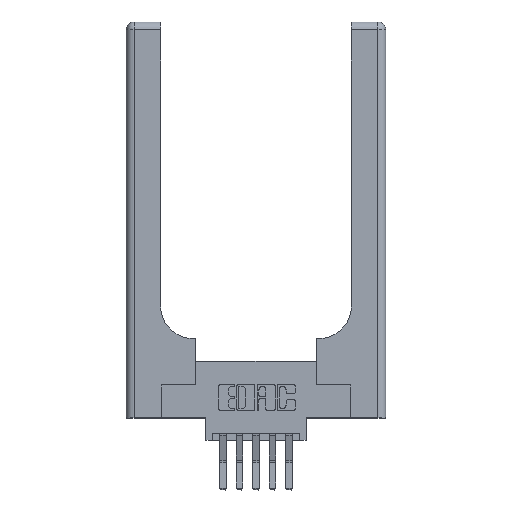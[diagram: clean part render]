
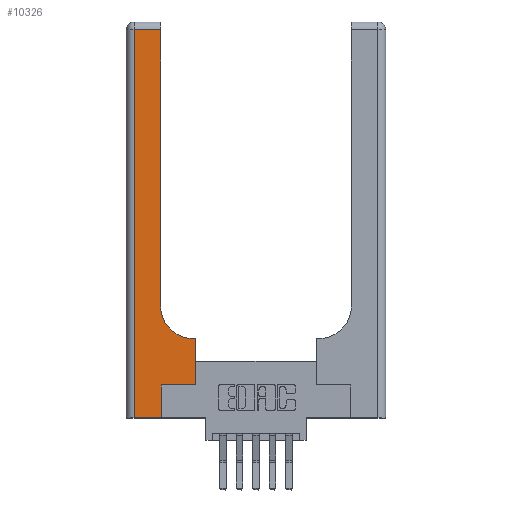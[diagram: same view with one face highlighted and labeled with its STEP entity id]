
A CAD part, top view. The second image highlights one B-rep face of the part: STEP entity #10326.
In plain terms, the highlighted planar face has unit normal (0, 0, 1).
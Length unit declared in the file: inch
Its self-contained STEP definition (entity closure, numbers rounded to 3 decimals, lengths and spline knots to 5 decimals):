
#12 = LINE ( 'NONE', #1932, #660 ) ;
#51 = CARTESIAN_POINT ( 'NONE',  ( 0., 3., 0.37 ) ) ;
#212 = CARTESIAN_POINT ( 'NONE',  ( 0.265, 0., 0.37 ) ) ;
#213 = VERTEX_POINT ( 'NONE', #4080 ) ;
#253 = LINE ( 'NONE', #3609, #4139 ) ;
#439 = LINE ( 'NONE', #8137, #5511 ) ;
#660 = VECTOR ( 'NONE', #1157, 39.37008 ) ;
#1089 = CARTESIAN_POINT ( 'NONE',  ( 0.265, 0.25, 0.37 ) ) ;
#1157 = DIRECTION ( 'NONE',  ( 1., 0., 0. ) ) ;
#1207 = ORIENTED_EDGE ( 'NONE', *, *, #13579, .T. ) ;
#1442 = CARTESIAN_POINT ( 'NONE',  ( 0.26, 0.85, 0.37 ) ) ;
#1565 = VERTEX_POINT ( 'NONE', #5509 ) ;
#1866 = CARTESIAN_POINT ( 'NONE',  ( 0.06, 2.94, 0.37 ) ) ;
#1932 = CARTESIAN_POINT ( 'NONE',  ( 0., 0., 0.37 ) ) ;
#1980 = EDGE_CURVE ( 'NONE', #1565, #7641, #12709, .T. ) ;
#2220 = DIRECTION ( 'NONE',  ( 1., 0., 0. ) ) ;
#2397 = ORIENTED_EDGE ( 'NONE', *, *, #9076, .T. ) ;
#2704 = CARTESIAN_POINT ( 'NONE',  ( 0.528, 0.25, 0.37 ) ) ;
#2726 = VECTOR ( 'NONE', #9642, 39.37008 ) ;
#2916 = CARTESIAN_POINT ( 'NONE',  ( 0.51, 0.6, 0.37 ) ) ;
#3021 = DIRECTION ( 'NONE',  ( 1., 0., 0. ) ) ;
#3124 = CARTESIAN_POINT ( 'NONE',  ( 0.26, 2.94, 0.37 ) ) ;
#3398 = ORIENTED_EDGE ( 'NONE', *, *, #11224, .T. ) ;
#3609 = CARTESIAN_POINT ( 'NONE',  ( 0.265, 0., 0.37 ) ) ;
#3997 = CARTESIAN_POINT ( 'NONE',  ( 0.51, 0.85, 0.37 ) ) ;
#4080 = CARTESIAN_POINT ( 'NONE',  ( 0.265, 0.25, 0.37 ) ) ;
#4139 = VECTOR ( 'NONE', #13433, 39.37008 ) ;
#4231 = LINE ( 'NONE', #13734, #12938 ) ;
#4383 = VERTEX_POINT ( 'NONE', #212 ) ;
#4385 = DIRECTION ( 'NONE',  ( 0., 0., -1. ) ) ;
#4417 = EDGE_CURVE ( 'NONE', #8698, #11114, #9402, .T. ) ;
#4444 = VERTEX_POINT ( 'NONE', #2704 ) ;
#4568 = VECTOR ( 'NONE', #2220, 39.37008 ) ;
#4759 = DIRECTION ( 'NONE',  ( -1., 0., 0. ) ) ;
#4948 = CIRCLE ( 'NONE', #11543, 0.25 ) ;
#5041 = ORIENTED_EDGE ( 'NONE', *, *, #1980, .T. ) ;
#5509 = CARTESIAN_POINT ( 'NONE',  ( 0.528, 0.6, 0.37 ) ) ;
#5511 = VECTOR ( 'NONE', #8068, 39.37008 ) ;
#5549 = EDGE_CURVE ( 'NONE', #7641, #5985, #4948, .T. ) ;
#5814 = ORIENTED_EDGE ( 'NONE', *, *, #5549, .T. ) ;
#5891 = VECTOR ( 'NONE', #6091, 39.37008 ) ;
#5985 = VERTEX_POINT ( 'NONE', #1442 ) ;
#6091 = DIRECTION ( 'NONE',  ( -1., 0., 0. ) ) ;
#7641 = VERTEX_POINT ( 'NONE', #2916 ) ;
#7745 = FACE_OUTER_BOUND ( 'NONE', #11684, .T. ) ;
#7810 = VERTEX_POINT ( 'NONE', #10107 ) ;
#8068 = DIRECTION ( 'NONE',  ( 0., -1., 0. ) ) ;
#8137 = CARTESIAN_POINT ( 'NONE',  ( 0.06, 3., 0.37 ) ) ;
#8162 = CARTESIAN_POINT ( 'NONE',  ( 0.26, 0.6, 0.37 ) ) ;
#8220 = DIRECTION ( 'NONE',  ( 0., 0., -1. ) ) ;
#8698 = VERTEX_POINT ( 'NONE', #3124 ) ;
#9076 = EDGE_CURVE ( 'NONE', #4444, #1565, #4231, .T. ) ;
#9253 = VECTOR ( 'NONE', #4759, 39.37008 ) ;
#9402 = LINE ( 'NONE', #13597, #9253 ) ;
#9479 = ORIENTED_EDGE ( 'NONE', *, *, #9546, .T. ) ;
#9546 = EDGE_CURVE ( 'NONE', #7810, #4383, #12, .T. ) ;
#9642 = DIRECTION ( 'NONE',  ( 0., 1., 0. ) ) ;
#9700 = ORIENTED_EDGE ( 'NONE', *, *, #14067, .T. ) ;
#9780 = CARTESIAN_POINT ( 'NONE',  ( 0.26, 3., 0.37 ) ) ;
#9787 = EDGE_CURVE ( 'NONE', #5985, #8698, #11871, .T. ) ;
#10107 = CARTESIAN_POINT ( 'NONE',  ( 0.06, 0., 0.37 ) ) ;
#10326 = ADVANCED_FACE ( 'NONE', ( #7745 ), #12068, .F. ) ;
#10729 = ORIENTED_EDGE ( 'NONE', *, *, #9787, .T. ) ;
#11114 = VERTEX_POINT ( 'NONE', #1866 ) ;
#11224 = EDGE_CURVE ( 'NONE', #213, #4444, #12292, .T. ) ;
#11543 = AXIS2_PLACEMENT_3D ( 'NONE', #3997, #8220, #3021 ) ;
#11684 = EDGE_LOOP ( 'NONE', ( #10729, #12800, #1207, #9479, #9700, #3398, #2397, #5041, #5814 ) ) ;
#11871 = LINE ( 'NONE', #9780, #2726 ) ;
#12068 = PLANE ( 'NONE',  #12267 ) ;
#12267 = AXIS2_PLACEMENT_3D ( 'NONE', #51, #4385, #13073 ) ;
#12292 = LINE ( 'NONE', #1089, #4568 ) ;
#12709 = LINE ( 'NONE', #8162, #5891 ) ;
#12800 = ORIENTED_EDGE ( 'NONE', *, *, #4417, .T. ) ;
#12929 = DIRECTION ( 'NONE',  ( 0., 1., 0. ) ) ;
#12938 = VECTOR ( 'NONE', #12929, 39.37008 ) ;
#13073 = DIRECTION ( 'NONE',  ( -1., 0., 0. ) ) ;
#13433 = DIRECTION ( 'NONE',  ( 0., 1., 0. ) ) ;
#13579 = EDGE_CURVE ( 'NONE', #11114, #7810, #439, .T. ) ;
#13597 = CARTESIAN_POINT ( 'NONE',  ( 0., 2.94, 0.37 ) ) ;
#13734 = CARTESIAN_POINT ( 'NONE',  ( 0.528, 0.25, 0.37 ) ) ;
#14067 = EDGE_CURVE ( 'NONE', #4383, #213, #253, .T. ) ;
